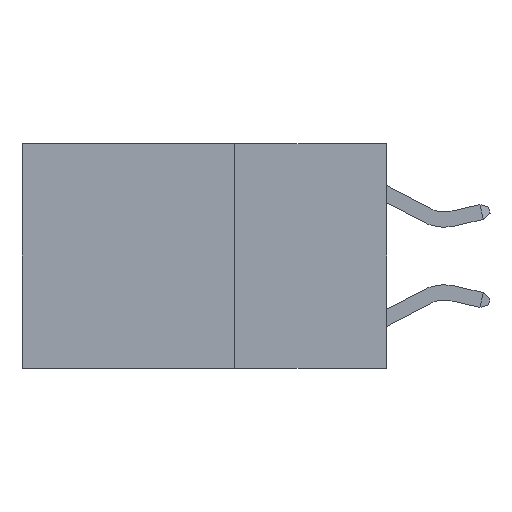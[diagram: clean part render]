
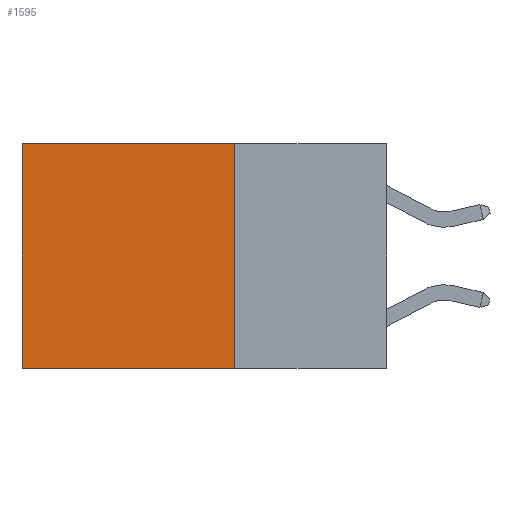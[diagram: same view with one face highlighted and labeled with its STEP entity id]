
A CAD part, left-side view. The second image highlights one B-rep face of the part: STEP entity #1595.
In plain terms, the highlighted planar face has unit normal (-1, 0, 0).
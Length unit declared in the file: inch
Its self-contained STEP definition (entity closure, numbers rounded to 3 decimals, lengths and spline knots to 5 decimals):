
#708 = AXIS2_PLACEMENT_3D ( 'NONE', #4329, #4160, #4099 ) ;
#1099 = VERTEX_POINT ( 'NONE', #13999 ) ;
#1515 = VERTEX_POINT ( 'NONE', #5480 ) ;
#1595 = ADVANCED_FACE ( 'NONE', ( #3456 ), #4525, .F. ) ;
#3084 = CARTESIAN_POINT ( 'NONE',  ( 0.2625, 0.25, 0. ) ) ;
#3363 = CARTESIAN_POINT ( 'NONE',  ( 0.2625, 0.25, -0.37 ) ) ;
#3409 = LINE ( 'NONE', #6120, #9259 ) ;
#3412 = ORIENTED_EDGE ( 'NONE', *, *, #6585, .T. ) ;
#3429 = LINE ( 'NONE', #8794, #9278 ) ;
#3456 = FACE_OUTER_BOUND ( 'NONE', #5929, .T. ) ;
#3692 = VECTOR ( 'NONE', #12503, 39.37008 ) ;
#4099 = DIRECTION ( 'NONE',  ( 0., 0., -1. ) ) ;
#4103 = ORIENTED_EDGE ( 'NONE', *, *, #8799, .T. ) ;
#4160 = DIRECTION ( 'NONE',  ( 1., 0., 0. ) ) ;
#4329 = CARTESIAN_POINT ( 'NONE',  ( 0.2625, 0.25, 0. ) ) ;
#4485 = ORIENTED_EDGE ( 'NONE', *, *, #6808, .F. ) ;
#4525 = PLANE ( 'NONE',  #708 ) ;
#4619 = CARTESIAN_POINT ( 'NONE',  ( 0.2625, 0.6, 0. ) ) ;
#4931 = DIRECTION ( 'NONE',  ( 0., 1., 0. ) ) ;
#5480 = CARTESIAN_POINT ( 'NONE',  ( 0.2625, 0.25, 0. ) ) ;
#5929 = EDGE_LOOP ( 'NONE', ( #4103, #4485, #12936, #3412 ) ) ;
#6120 = CARTESIAN_POINT ( 'NONE',  ( 0.2625, 0.25, 0. ) ) ;
#6585 = EDGE_CURVE ( 'NONE', #1515, #10928, #3409, .T. ) ;
#6808 = EDGE_CURVE ( 'NONE', #14633, #1099, #3429, .T. ) ;
#7619 = DIRECTION ( 'NONE',  ( 0., 1., 0. ) ) ;
#8794 = CARTESIAN_POINT ( 'NONE',  ( 0.2625, 0.25, -0.37 ) ) ;
#8799 = EDGE_CURVE ( 'NONE', #10928, #1099, #12524, .T. ) ;
#9259 = VECTOR ( 'NONE', #4931, 39.37008 ) ;
#9278 = VECTOR ( 'NONE', #7619, 39.37008 ) ;
#9387 = VECTOR ( 'NONE', #13984, 39.37008 ) ;
#10275 = LINE ( 'NONE', #3084, #3692 ) ;
#10928 = VERTEX_POINT ( 'NONE', #13971 ) ;
#12503 = DIRECTION ( 'NONE',  ( 0., 0., -1. ) ) ;
#12524 = LINE ( 'NONE', #4619, #9387 ) ;
#12715 = EDGE_CURVE ( 'NONE', #1515, #14633, #10275, .T. ) ;
#12936 = ORIENTED_EDGE ( 'NONE', *, *, #12715, .F. ) ;
#13971 = CARTESIAN_POINT ( 'NONE',  ( 0.2625, 0.6, 0. ) ) ;
#13984 = DIRECTION ( 'NONE',  ( 0., 0., -1. ) ) ;
#13999 = CARTESIAN_POINT ( 'NONE',  ( 0.2625, 0.6, -0.37 ) ) ;
#14633 = VERTEX_POINT ( 'NONE', #3363 ) ;
